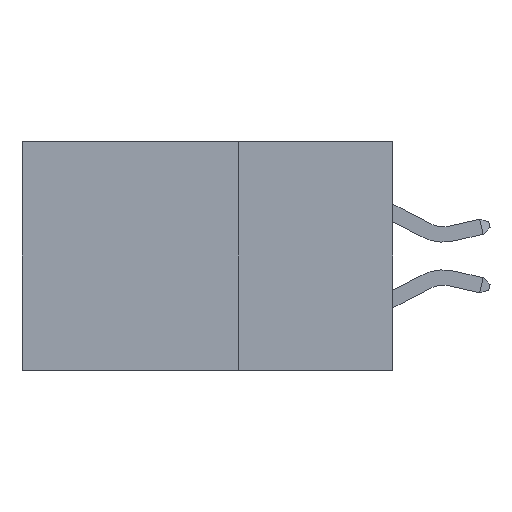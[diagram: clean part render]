
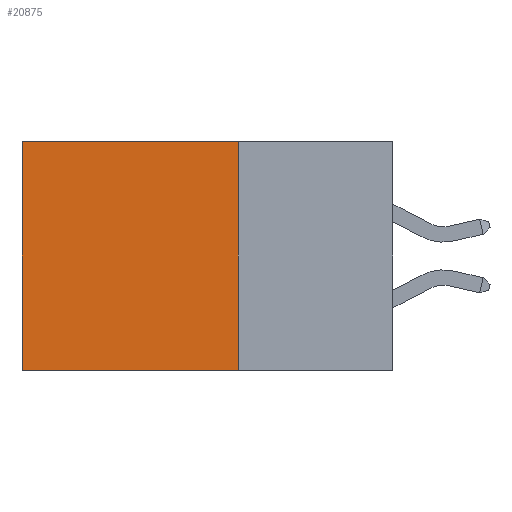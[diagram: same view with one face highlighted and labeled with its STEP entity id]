
A CAD part, left-side view. The second image highlights one B-rep face of the part: STEP entity #20875.
In plain terms, the highlighted planar face has unit normal (-1, 0, 0).
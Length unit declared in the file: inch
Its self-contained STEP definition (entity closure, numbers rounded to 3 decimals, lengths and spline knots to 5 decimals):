
#53 = EDGE_CURVE ( 'NONE', #19195, #14538, #2431, .T. ) ;
#359 = AXIS2_PLACEMENT_3D ( 'NONE', #1018, #19914, #9680 ) ;
#1018 = CARTESIAN_POINT ( 'NONE',  ( 0.2875, 0.25, 0. ) ) ;
#1093 = PLANE ( 'NONE',  #359 ) ;
#1379 = LINE ( 'NONE', #9968, #18914 ) ;
#1965 = DIRECTION ( 'NONE',  ( 0., 1., 0. ) ) ;
#2431 = LINE ( 'NONE', #21681, #4003 ) ;
#3978 = VERTEX_POINT ( 'NONE', #14523 ) ;
#4003 = VECTOR ( 'NONE', #18322, 39.37008 ) ;
#5414 = ORIENTED_EDGE ( 'NONE', *, *, #19665, .F. ) ;
#6218 = EDGE_LOOP ( 'NONE', ( #15983, #5414, #21888, #18547 ) ) ;
#6763 = VECTOR ( 'NONE', #20959, 39.37008 ) ;
#9651 = DIRECTION ( 'NONE',  ( 0., 1., 0. ) ) ;
#9680 = DIRECTION ( 'NONE',  ( 0., 0., -1. ) ) ;
#9968 = CARTESIAN_POINT ( 'NONE',  ( 0.2875, 0.25, 0. ) ) ;
#11470 = EDGE_CURVE ( 'NONE', #3978, #14552, #15357, .T. ) ;
#12445 = CARTESIAN_POINT ( 'NONE',  ( 0.2875, 0.6, -0.37 ) ) ;
#13772 = FACE_OUTER_BOUND ( 'NONE', #6218, .T. ) ;
#14523 = CARTESIAN_POINT ( 'NONE',  ( 0.2875, 0.6, 0. ) ) ;
#14538 = VERTEX_POINT ( 'NONE', #21019 ) ;
#14552 = VERTEX_POINT ( 'NONE', #12445 ) ;
#14651 = VECTOR ( 'NONE', #9651, 39.37008 ) ;
#15357 = LINE ( 'NONE', #16148, #6763 ) ;
#15983 = ORIENTED_EDGE ( 'NONE', *, *, #11470, .T. ) ;
#16148 = CARTESIAN_POINT ( 'NONE',  ( 0.2875, 0.6, 0. ) ) ;
#16398 = CARTESIAN_POINT ( 'NONE',  ( 0.2875, 0.25, -0.37 ) ) ;
#18322 = DIRECTION ( 'NONE',  ( 0., 0., -1. ) ) ;
#18547 = ORIENTED_EDGE ( 'NONE', *, *, #19248, .T. ) ;
#18914 = VECTOR ( 'NONE', #1965, 39.37008 ) ;
#19195 = VERTEX_POINT ( 'NONE', #20353 ) ;
#19248 = EDGE_CURVE ( 'NONE', #19195, #3978, #1379, .T. ) ;
#19665 = EDGE_CURVE ( 'NONE', #14538, #14552, #19712, .T. ) ;
#19712 = LINE ( 'NONE', #16398, #14651 ) ;
#19914 = DIRECTION ( 'NONE',  ( 1., 0., 0. ) ) ;
#20353 = CARTESIAN_POINT ( 'NONE',  ( 0.2875, 0.25, 0. ) ) ;
#20875 = ADVANCED_FACE ( 'NONE', ( #13772 ), #1093, .F. ) ;
#20959 = DIRECTION ( 'NONE',  ( 0., 0., -1. ) ) ;
#21019 = CARTESIAN_POINT ( 'NONE',  ( 0.2875, 0.25, -0.37 ) ) ;
#21681 = CARTESIAN_POINT ( 'NONE',  ( 0.2875, 0.25, 0. ) ) ;
#21888 = ORIENTED_EDGE ( 'NONE', *, *, #53, .F. ) ;
